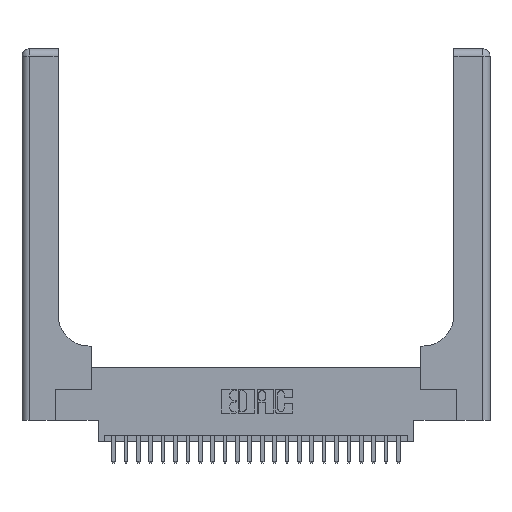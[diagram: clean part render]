
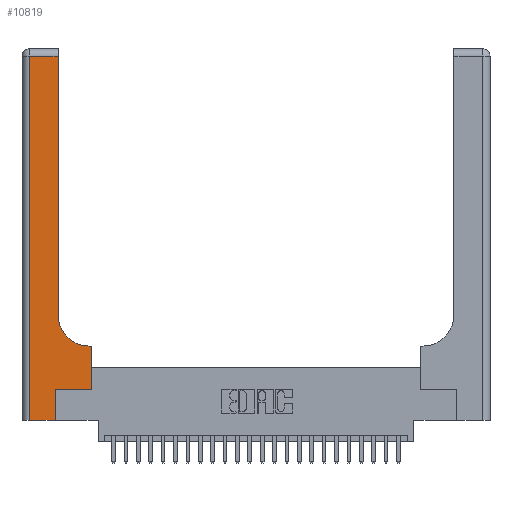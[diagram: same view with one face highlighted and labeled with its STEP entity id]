
A CAD part, top view. The second image highlights one B-rep face of the part: STEP entity #10819.
In plain terms, the highlighted planar face has unit normal (0, 0, 1).
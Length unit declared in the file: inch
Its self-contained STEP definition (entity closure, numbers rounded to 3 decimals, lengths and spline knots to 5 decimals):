
#111 = ORIENTED_EDGE ( 'NONE', *, *, #9021, .T. ) ;
#114 = CARTESIAN_POINT ( 'NONE',  ( 0.5415, 0.85, 0.37 ) ) ;
#418 = VECTOR ( 'NONE', #24461, 39.37008 ) ;
#1031 = CARTESIAN_POINT ( 'NONE',  ( 0., 3., 0.37 ) ) ;
#1048 = VERTEX_POINT ( 'NONE', #5015 ) ;
#1452 = EDGE_CURVE ( 'NONE', #1048, #7383, #10687, .T. ) ;
#1484 = VECTOR ( 'NONE', #24029, 39.37008 ) ;
#1719 = DIRECTION ( 'NONE',  ( 0., 1., 0. ) ) ;
#1815 = EDGE_CURVE ( 'NONE', #19980, #1048, #5209, .T. ) ;
#2290 = VERTEX_POINT ( 'NONE', #15239 ) ;
#2620 = CARTESIAN_POINT ( 'NONE',  ( 0.2915, 2.94, 0.37 ) ) ;
#3023 = DIRECTION ( 'NONE',  ( -1., 0., 0. ) ) ;
#3481 = DIRECTION ( 'NONE',  ( 0., -1., 0. ) ) ;
#3529 = CARTESIAN_POINT ( 'NONE',  ( 0.269, 0., 0.37 ) ) ;
#3935 = VERTEX_POINT ( 'NONE', #24763 ) ;
#4025 = VECTOR ( 'NONE', #10805, 39.37008 ) ;
#4665 = LINE ( 'NONE', #15129, #4025 ) ;
#4884 = VECTOR ( 'NONE', #12310, 39.37008 ) ;
#5015 = CARTESIAN_POINT ( 'NONE',  ( 0.5415, 0.6, 0.37 ) ) ;
#5209 = LINE ( 'NONE', #24931, #4884 ) ;
#5304 = VERTEX_POINT ( 'NONE', #13642 ) ;
#6236 = VECTOR ( 'NONE', #26563, 39.37008 ) ;
#6361 = DIRECTION ( 'NONE',  ( 0., 0., -1. ) ) ;
#7003 = LINE ( 'NONE', #26105, #1484 ) ;
#7116 = DIRECTION ( 'NONE',  ( 0., 0., -1. ) ) ;
#7383 = VERTEX_POINT ( 'NONE', #9635 ) ;
#7480 = EDGE_CURVE ( 'NONE', #19281, #5304, #7003, .T. ) ;
#9021 = EDGE_CURVE ( 'NONE', #3935, #19980, #19796, .T. ) ;
#9537 = CARTESIAN_POINT ( 'NONE',  ( 0.06, 3., 0.37 ) ) ;
#9635 = CARTESIAN_POINT ( 'NONE',  ( 0.2915, 0.85, 0.37 ) ) ;
#9879 = EDGE_LOOP ( 'NONE', ( #22603, #19889, #25529, #24492, #15534, #21991, #111, #14926, #20126 ) ) ;
#10274 = FACE_OUTER_BOUND ( 'NONE', #9879, .T. ) ;
#10687 = CIRCLE ( 'NONE', #11630, 0.25 ) ;
#10805 = DIRECTION ( 'NONE',  ( 0., 1., 0. ) ) ;
#10819 = ADVANCED_FACE ( 'NONE', ( #10274 ), #25989, .F. ) ;
#10969 = EDGE_CURVE ( 'NONE', #5304, #24677, #18945, .T. ) ;
#11452 = CARTESIAN_POINT ( 'NONE',  ( 0.06, 0., 0.37 ) ) ;
#11512 = VECTOR ( 'NONE', #3481, 39.37008 ) ;
#11630 = AXIS2_PLACEMENT_3D ( 'NONE', #114, #6361, #12628 ) ;
#12310 = DIRECTION ( 'NONE',  ( -1., 0., 0. ) ) ;
#12628 = DIRECTION ( 'NONE',  ( 1., 0., 0. ) ) ;
#13034 = CARTESIAN_POINT ( 'NONE',  ( 0.5585, 0.6, 0.37 ) ) ;
#13562 = DIRECTION ( 'NONE',  ( 1., 0., 0. ) ) ;
#13642 = CARTESIAN_POINT ( 'NONE',  ( 0.06, 2.94, 0.37 ) ) ;
#14926 = ORIENTED_EDGE ( 'NONE', *, *, #1815, .T. ) ;
#15129 = CARTESIAN_POINT ( 'NONE',  ( 0.2915, 3., 0.37 ) ) ;
#15239 = CARTESIAN_POINT ( 'NONE',  ( 0.269, 0.25, 0.37 ) ) ;
#15400 = CARTESIAN_POINT ( 'NONE',  ( 0.269, 0., 0.37 ) ) ;
#15534 = ORIENTED_EDGE ( 'NONE', *, *, #24795, .T. ) ;
#15803 = EDGE_CURVE ( 'NONE', #2290, #3935, #26106, .T. ) ;
#16405 = AXIS2_PLACEMENT_3D ( 'NONE', #1031, #7116, #3023 ) ;
#17530 = VECTOR ( 'NONE', #1719, 39.37008 ) ;
#17947 = EDGE_CURVE ( 'NONE', #24677, #25191, #25247, .T. ) ;
#18693 = VECTOR ( 'NONE', #13562, 39.37008 ) ;
#18945 = LINE ( 'NONE', #9537, #11512 ) ;
#19281 = VERTEX_POINT ( 'NONE', #2620 ) ;
#19796 = LINE ( 'NONE', #24402, #6236 ) ;
#19889 = ORIENTED_EDGE ( 'NONE', *, *, #7480, .T. ) ;
#19890 = CARTESIAN_POINT ( 'NONE',  ( 0.269, 0.25, 0.37 ) ) ;
#19980 = VERTEX_POINT ( 'NONE', #13034 ) ;
#20126 = ORIENTED_EDGE ( 'NONE', *, *, #1452, .T. ) ;
#21991 = ORIENTED_EDGE ( 'NONE', *, *, #15803, .T. ) ;
#22603 = ORIENTED_EDGE ( 'NONE', *, *, #23796, .T. ) ;
#23008 = LINE ( 'NONE', #3529, #17530 ) ;
#23796 = EDGE_CURVE ( 'NONE', #7383, #19281, #4665, .T. ) ;
#24029 = DIRECTION ( 'NONE',  ( -1., 0., 0. ) ) ;
#24402 = CARTESIAN_POINT ( 'NONE',  ( 0.5585, 0.25, 0.37 ) ) ;
#24461 = DIRECTION ( 'NONE',  ( 1., 0., 0. ) ) ;
#24492 = ORIENTED_EDGE ( 'NONE', *, *, #17947, .T. ) ;
#24677 = VERTEX_POINT ( 'NONE', #11452 ) ;
#24763 = CARTESIAN_POINT ( 'NONE',  ( 0.5585, 0.25, 0.37 ) ) ;
#24795 = EDGE_CURVE ( 'NONE', #25191, #2290, #23008, .T. ) ;
#24931 = CARTESIAN_POINT ( 'NONE',  ( 0.2915, 0.6, 0.37 ) ) ;
#24940 = CARTESIAN_POINT ( 'NONE',  ( 0., 0., 0.37 ) ) ;
#25191 = VERTEX_POINT ( 'NONE', #15400 ) ;
#25247 = LINE ( 'NONE', #24940, #418 ) ;
#25529 = ORIENTED_EDGE ( 'NONE', *, *, #10969, .T. ) ;
#25989 = PLANE ( 'NONE',  #16405 ) ;
#26105 = CARTESIAN_POINT ( 'NONE',  ( 0., 2.94, 0.37 ) ) ;
#26106 = LINE ( 'NONE', #19890, #18693 ) ;
#26563 = DIRECTION ( 'NONE',  ( 0., 1., 0. ) ) ;
